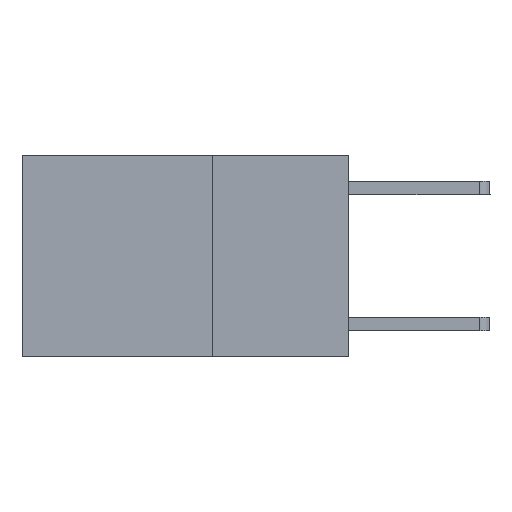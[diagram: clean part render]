
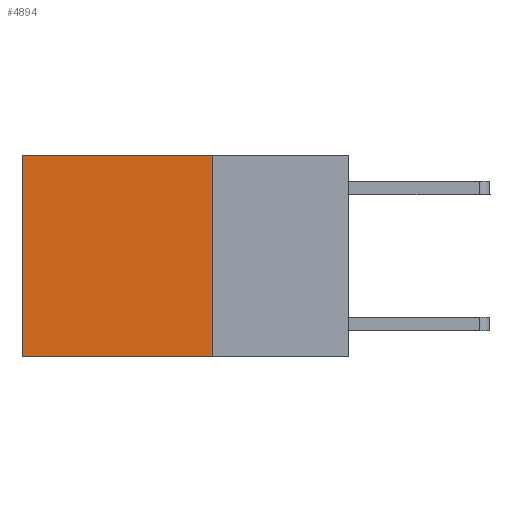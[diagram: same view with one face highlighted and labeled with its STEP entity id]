
A CAD part, left-side view. The second image highlights one B-rep face of the part: STEP entity #4894.
In plain terms, the highlighted planar face has unit normal (-1, 0, 0).
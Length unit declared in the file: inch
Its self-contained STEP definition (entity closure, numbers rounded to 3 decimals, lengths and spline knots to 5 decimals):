
#151 = EDGE_CURVE ( 'NONE', #5354, #5272, #1018, .T. ) ;
#379 = DIRECTION ( 'NONE',  ( 0., 0., -1. ) ) ;
#721 = LINE ( 'NONE', #3179, #9397 ) ;
#858 = EDGE_LOOP ( 'NONE', ( #6273, #6280, #6307, #6340 ) ) ;
#1018 = LINE ( 'NONE', #5709, #5581 ) ;
#1288 = EDGE_CURVE ( 'NONE', #10359, #5354, #3011, .T. ) ;
#1484 = CARTESIAN_POINT ( 'NONE',  ( 0.2625, 0.25, 0. ) ) ;
#1635 = VERTEX_POINT ( 'NONE', #10684 ) ;
#1787 = CARTESIAN_POINT ( 'NONE',  ( 0.2625, 0.6, 0. ) ) ;
#2423 = CARTESIAN_POINT ( 'NONE',  ( 0.2625, 0.6, -0.37 ) ) ;
#2835 = AXIS2_PLACEMENT_3D ( 'NONE', #7548, #5860, #379 ) ;
#3011 = LINE ( 'NONE', #6927, #7208 ) ;
#3179 = CARTESIAN_POINT ( 'NONE',  ( 0.2625, 0.25, 0. ) ) ;
#3213 = EDGE_CURVE ( 'NONE', #1635, #5272, #3869, .T. ) ;
#3869 = LINE ( 'NONE', #7481, #8305 ) ;
#3992 = DIRECTION ( 'NONE',  ( 0., 0., -1. ) ) ;
#4855 = FACE_OUTER_BOUND ( 'NONE', #858, .T. ) ;
#4867 = PLANE ( 'NONE',  #2835 ) ;
#4894 = ADVANCED_FACE ( 'NONE', ( #4855 ), #4867, .F. ) ;
#5272 = VERTEX_POINT ( 'NONE', #2423 ) ;
#5354 = VERTEX_POINT ( 'NONE', #1787 ) ;
#5581 = VECTOR ( 'NONE', #7562, 39.37008 ) ;
#5709 = CARTESIAN_POINT ( 'NONE',  ( 0.2625, 0.6, 0. ) ) ;
#5860 = DIRECTION ( 'NONE',  ( 1., 0., 0. ) ) ;
#6259 = DIRECTION ( 'NONE',  ( 0., 1., 0. ) ) ;
#6273 = ORIENTED_EDGE ( 'NONE', *, *, #151, .T. ) ;
#6280 = ORIENTED_EDGE ( 'NONE', *, *, #3213, .F. ) ;
#6307 = ORIENTED_EDGE ( 'NONE', *, *, #6676, .F. ) ;
#6340 = ORIENTED_EDGE ( 'NONE', *, *, #1288, .T. ) ;
#6676 = EDGE_CURVE ( 'NONE', #10359, #1635, #721, .T. ) ;
#6927 = CARTESIAN_POINT ( 'NONE',  ( 0.2625, 0.25, 0. ) ) ;
#7208 = VECTOR ( 'NONE', #6259, 39.37008 ) ;
#7481 = CARTESIAN_POINT ( 'NONE',  ( 0.2625, 0.25, -0.37 ) ) ;
#7548 = CARTESIAN_POINT ( 'NONE',  ( 0.2625, 0.25, 0. ) ) ;
#7562 = DIRECTION ( 'NONE',  ( 0., 0., -1. ) ) ;
#8305 = VECTOR ( 'NONE', #9023, 39.37008 ) ;
#9023 = DIRECTION ( 'NONE',  ( 0., 1., 0. ) ) ;
#9397 = VECTOR ( 'NONE', #3992, 39.37008 ) ;
#10359 = VERTEX_POINT ( 'NONE', #1484 ) ;
#10684 = CARTESIAN_POINT ( 'NONE',  ( 0.2625, 0.25, -0.37 ) ) ;
